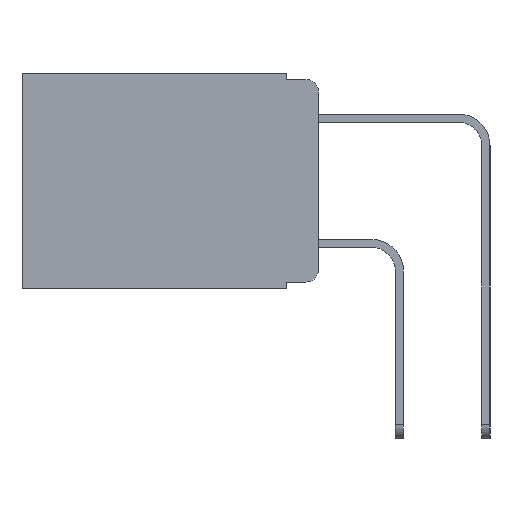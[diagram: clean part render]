
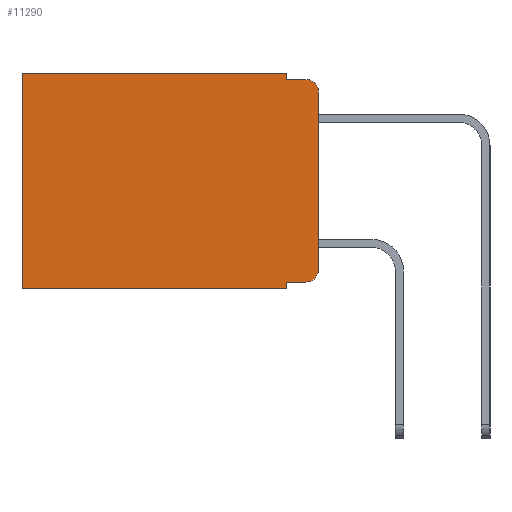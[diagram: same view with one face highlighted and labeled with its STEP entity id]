
A CAD part, left-side view. The second image highlights one B-rep face of the part: STEP entity #11290.
In plain terms, the highlighted planar face has unit normal (-1, 0, 0).
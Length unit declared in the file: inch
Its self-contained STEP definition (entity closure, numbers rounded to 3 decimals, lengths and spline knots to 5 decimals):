
#62 = VERTEX_POINT ( 'NONE', #2344 ) ;
#459 = ORIENTED_EDGE ( 'NONE', *, *, #11360, .T. ) ;
#477 = ORIENTED_EDGE ( 'NONE', *, *, #7231, .F. ) ;
#521 = ORIENTED_EDGE ( 'NONE', *, *, #8705, .F. ) ;
#671 = CARTESIAN_POINT ( 'NONE',  ( 0.298, 0.051, -0.333 ) ) ;
#761 = ORIENTED_EDGE ( 'NONE', *, *, #5868, .T. ) ;
#990 = LINE ( 'NONE', #9842, #6381 ) ;
#1010 = CARTESIAN_POINT ( 'NONE',  ( 0.298, 0.02, -0.01 ) ) ;
#1110 = ORIENTED_EDGE ( 'NONE', *, *, #7884, .F. ) ;
#1453 = ORIENTED_EDGE ( 'NONE', *, *, #10397, .F. ) ;
#1500 = CARTESIAN_POINT ( 'NONE',  ( 0.298, 0.051, 0. ) ) ;
#1522 = CIRCLE ( 'NONE', #6581, 0.02 ) ;
#1523 = CARTESIAN_POINT ( 'NONE',  ( 0.298, 0.473, 0. ) ) ;
#1562 = LINE ( 'NONE', #10213, #4179 ) ;
#1962 = EDGE_LOOP ( 'NONE', ( #1453, #2262, #1110, #477, #459, #761, #521, #7687, #7829, #2122 ) ) ;
#1969 = CARTESIAN_POINT ( 'NONE',  ( 0.298, 0.473, 0. ) ) ;
#2122 = ORIENTED_EDGE ( 'NONE', *, *, #3067, .T. ) ;
#2262 = ORIENTED_EDGE ( 'NONE', *, *, #8534, .T. ) ;
#2344 = CARTESIAN_POINT ( 'NONE',  ( 0.298, 0.051, -0.343 ) ) ;
#2633 = VERTEX_POINT ( 'NONE', #671 ) ;
#2643 = DIRECTION ( 'NONE',  ( -1., 0., 0. ) ) ;
#3067 = EDGE_CURVE ( 'NONE', #11372, #3391, #1522, .T. ) ;
#3072 = CARTESIAN_POINT ( 'NONE',  ( 0.298, 0., -0.03 ) ) ;
#3276 = VERTEX_POINT ( 'NONE', #1969 ) ;
#3352 = CARTESIAN_POINT ( 'NONE',  ( 0.298, 0., 0. ) ) ;
#3391 = VERTEX_POINT ( 'NONE', #13070 ) ;
#3680 = DIRECTION ( 'NONE',  ( -1., 0., 0. ) ) ;
#3804 = EDGE_CURVE ( 'NONE', #2633, #11372, #9964, .T. ) ;
#3859 = VERTEX_POINT ( 'NONE', #7076 ) ;
#4129 = VECTOR ( 'NONE', #8904, 39.37008 ) ;
#4179 = VECTOR ( 'NONE', #6405, 39.37008 ) ;
#4593 = VECTOR ( 'NONE', #12405, 39.37008 ) ;
#5201 = EDGE_CURVE ( 'NONE', #2633, #62, #8924, .T. ) ;
#5273 = CIRCLE ( 'NONE', #10933, 0.02 ) ;
#5465 = DIRECTION ( 'NONE',  ( 1., 0., 0. ) ) ;
#5627 = CARTESIAN_POINT ( 'NONE',  ( 0.298, 0., 0. ) ) ;
#5805 = LINE ( 'NONE', #1523, #8154 ) ;
#5868 = EDGE_CURVE ( 'NONE', #3276, #8470, #5805, .T. ) ;
#5993 = VECTOR ( 'NONE', #10550, 39.37008 ) ;
#6381 = VECTOR ( 'NONE', #7999, 39.37008 ) ;
#6405 = DIRECTION ( 'NONE',  ( 0., 0., -1. ) ) ;
#6441 = PLANE ( 'NONE',  #8275 ) ;
#6502 = FACE_OUTER_BOUND ( 'NONE', #1962, .T. ) ;
#6581 = AXIS2_PLACEMENT_3D ( 'NONE', #11487, #3680, #10572 ) ;
#6853 = LINE ( 'NONE', #12624, #4129 ) ;
#7076 = CARTESIAN_POINT ( 'NONE',  ( 0.298, 0.051, -0.01 ) ) ;
#7119 = VERTEX_POINT ( 'NONE', #3072 ) ;
#7231 = EDGE_CURVE ( 'NONE', #12217, #3859, #1562, .T. ) ;
#7271 = LINE ( 'NONE', #5627, #4593 ) ;
#7687 = ORIENTED_EDGE ( 'NONE', *, *, #5201, .F. ) ;
#7829 = ORIENTED_EDGE ( 'NONE', *, *, #3804, .T. ) ;
#7884 = EDGE_CURVE ( 'NONE', #3859, #12434, #11032, .T. ) ;
#7999 = DIRECTION ( 'NONE',  ( 0., 1., 0. ) ) ;
#8065 = VECTOR ( 'NONE', #11203, 39.37008 ) ;
#8097 = CARTESIAN_POINT ( 'NONE',  ( 0.298, 0.051, -0.01 ) ) ;
#8154 = VECTOR ( 'NONE', #8795, 39.37008 ) ;
#8275 = AXIS2_PLACEMENT_3D ( 'NONE', #3352, #5465, #12238 ) ;
#8470 = VERTEX_POINT ( 'NONE', #8634 ) ;
#8534 = EDGE_CURVE ( 'NONE', #7119, #12434, #5273, .T. ) ;
#8554 = VECTOR ( 'NONE', #10926, 39.37008 ) ;
#8634 = CARTESIAN_POINT ( 'NONE',  ( 0.298, 0.473, -0.343 ) ) ;
#8705 = EDGE_CURVE ( 'NONE', #62, #8470, #990, .T. ) ;
#8760 = CARTESIAN_POINT ( 'NONE',  ( 0.298, 0.051, -0.333 ) ) ;
#8769 = CARTESIAN_POINT ( 'NONE',  ( 0.298, 0.02, -0.03 ) ) ;
#8795 = DIRECTION ( 'NONE',  ( 0., 0., -1. ) ) ;
#8904 = DIRECTION ( 'NONE',  ( 0., 0., -1. ) ) ;
#8924 = LINE ( 'NONE', #12503, #5993 ) ;
#9687 = DIRECTION ( 'NONE',  ( 0., 0., -1. ) ) ;
#9842 = CARTESIAN_POINT ( 'NONE',  ( 0.298, 0., -0.343 ) ) ;
#9964 = LINE ( 'NONE', #8760, #8065 ) ;
#10213 = CARTESIAN_POINT ( 'NONE',  ( 0.298, 0.051, 0. ) ) ;
#10397 = EDGE_CURVE ( 'NONE', #7119, #3391, #6853, .T. ) ;
#10550 = DIRECTION ( 'NONE',  ( 0., 0., -1. ) ) ;
#10572 = DIRECTION ( 'NONE',  ( 0., 0., -1. ) ) ;
#10926 = DIRECTION ( 'NONE',  ( 0., -1., 0. ) ) ;
#10933 = AXIS2_PLACEMENT_3D ( 'NONE', #8769, #2643, #9687 ) ;
#11032 = LINE ( 'NONE', #8097, #8554 ) ;
#11203 = DIRECTION ( 'NONE',  ( 0., -1., 0. ) ) ;
#11290 = ADVANCED_FACE ( 'NONE', ( #6502 ), #6441, .F. ) ;
#11360 = EDGE_CURVE ( 'NONE', #12217, #3276, #7271, .T. ) ;
#11372 = VERTEX_POINT ( 'NONE', #11401 ) ;
#11401 = CARTESIAN_POINT ( 'NONE',  ( 0.298, 0.02, -0.333 ) ) ;
#11487 = CARTESIAN_POINT ( 'NONE',  ( 0.298, 0.02, -0.313 ) ) ;
#12217 = VERTEX_POINT ( 'NONE', #1500 ) ;
#12238 = DIRECTION ( 'NONE',  ( 0., 0., -1. ) ) ;
#12405 = DIRECTION ( 'NONE',  ( 0., 1., 0. ) ) ;
#12434 = VERTEX_POINT ( 'NONE', #1010 ) ;
#12503 = CARTESIAN_POINT ( 'NONE',  ( 0.298, 0.051, 0. ) ) ;
#12624 = CARTESIAN_POINT ( 'NONE',  ( 0.298, 0., 0. ) ) ;
#13070 = CARTESIAN_POINT ( 'NONE',  ( 0.298, 0., -0.313 ) ) ;
